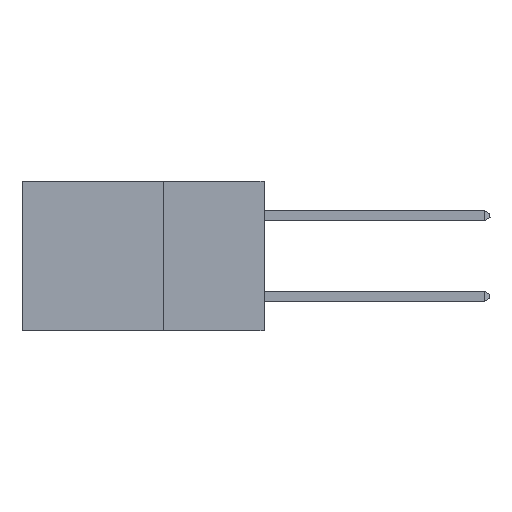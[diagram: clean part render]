
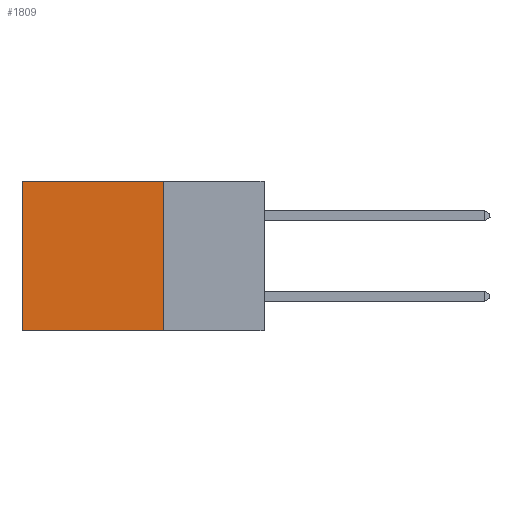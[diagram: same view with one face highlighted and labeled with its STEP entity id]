
A CAD part, left-side view. The second image highlights one B-rep face of the part: STEP entity #1809.
In plain terms, the highlighted planar face has unit normal (-1, 0, 0).
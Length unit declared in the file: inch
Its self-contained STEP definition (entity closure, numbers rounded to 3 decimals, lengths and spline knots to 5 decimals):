
#1075 = ORIENTED_EDGE ( 'NONE', *, *, #7236, .F. ) ;
#1121 = CARTESIAN_POINT ( 'NONE',  ( 0.298, 0.6, -0.37 ) ) ;
#1459 = VERTEX_POINT ( 'NONE', #1121 ) ;
#1584 = DIRECTION ( 'NONE',  ( 0., 0., -1. ) ) ;
#1725 = LINE ( 'NONE', #12771, #4938 ) ;
#1809 = ADVANCED_FACE ( 'NONE', ( #7912 ), #16001, .F. ) ;
#2489 = VECTOR ( 'NONE', #1584, 39.37008 ) ;
#3057 = CARTESIAN_POINT ( 'NONE',  ( 0.298, 0.25, 0. ) ) ;
#4565 = LINE ( 'NONE', #13579, #17434 ) ;
#4938 = VECTOR ( 'NONE', #15619, 39.37008 ) ;
#5869 = EDGE_CURVE ( 'NONE', #14617, #13524, #7890, .T. ) ;
#6118 = LINE ( 'NONE', #11080, #2489 ) ;
#6287 = EDGE_LOOP ( 'NONE', ( #14338, #1075, #10194, #12481 ) ) ;
#6440 = DIRECTION ( 'NONE',  ( 0., 0., -1. ) ) ;
#6630 = CARTESIAN_POINT ( 'NONE',  ( 0.298, 0.6, 0. ) ) ;
#6742 = EDGE_CURVE ( 'NONE', #13241, #1459, #6118, .T. ) ;
#7236 = EDGE_CURVE ( 'NONE', #13524, #1459, #4565, .T. ) ;
#7890 = LINE ( 'NONE', #17429, #16444 ) ;
#7912 = FACE_OUTER_BOUND ( 'NONE', #6287, .T. ) ;
#10194 = ORIENTED_EDGE ( 'NONE', *, *, #5869, .F. ) ;
#10539 = DIRECTION ( 'NONE',  ( 1., 0., 0. ) ) ;
#11080 = CARTESIAN_POINT ( 'NONE',  ( 0.298, 0.6, 0. ) ) ;
#11936 = DIRECTION ( 'NONE',  ( 0., 0., -1. ) ) ;
#12481 = ORIENTED_EDGE ( 'NONE', *, *, #12973, .T. ) ;
#12771 = CARTESIAN_POINT ( 'NONE',  ( 0.298, 0.25, 0. ) ) ;
#12973 = EDGE_CURVE ( 'NONE', #14617, #13241, #1725, .T. ) ;
#13241 = VERTEX_POINT ( 'NONE', #6630 ) ;
#13524 = VERTEX_POINT ( 'NONE', #17122 ) ;
#13579 = CARTESIAN_POINT ( 'NONE',  ( 0.298, 0.25, -0.37 ) ) ;
#13818 = DIRECTION ( 'NONE',  ( 0., 1., 0. ) ) ;
#14338 = ORIENTED_EDGE ( 'NONE', *, *, #6742, .T. ) ;
#14617 = VERTEX_POINT ( 'NONE', #3057 ) ;
#15058 = AXIS2_PLACEMENT_3D ( 'NONE', #17103, #10539, #11936 ) ;
#15619 = DIRECTION ( 'NONE',  ( 0., 1., 0. ) ) ;
#16001 = PLANE ( 'NONE',  #15058 ) ;
#16444 = VECTOR ( 'NONE', #6440, 39.37008 ) ;
#17103 = CARTESIAN_POINT ( 'NONE',  ( 0.298, 0.25, 0. ) ) ;
#17122 = CARTESIAN_POINT ( 'NONE',  ( 0.298, 0.25, -0.37 ) ) ;
#17429 = CARTESIAN_POINT ( 'NONE',  ( 0.298, 0.25, 0. ) ) ;
#17434 = VECTOR ( 'NONE', #13818, 39.37008 ) ;
